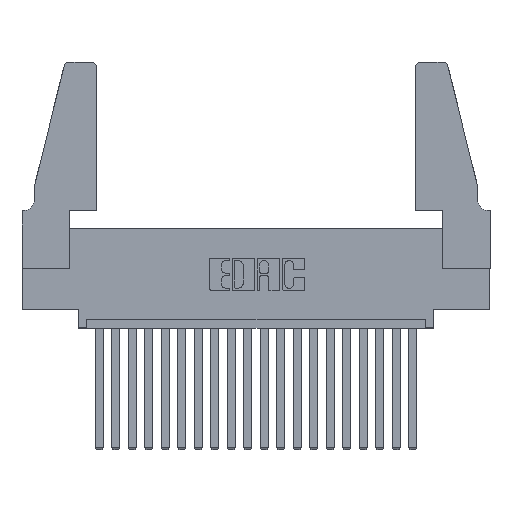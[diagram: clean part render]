
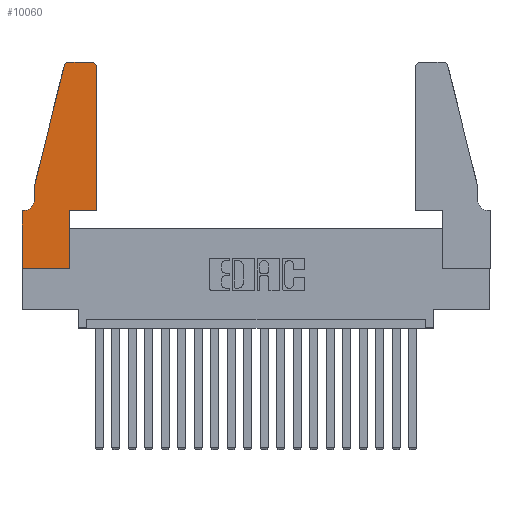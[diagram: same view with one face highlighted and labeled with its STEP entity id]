
A CAD part, top view. The second image highlights one B-rep face of the part: STEP entity #10060.
In plain terms, the highlighted planar face has unit normal (0, 0, 1).
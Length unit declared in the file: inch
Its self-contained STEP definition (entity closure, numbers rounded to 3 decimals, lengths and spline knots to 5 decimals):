
#19 = CARTESIAN_POINT ( 'NONE',  ( 0.0055, 0.42, 0.37 ) ) ;
#578 = CARTESIAN_POINT ( 'NONE',  ( 0.0055, 0.35, 0.37 ) ) ;
#1022 = VECTOR ( 'NONE', #19834, 39.37008 ) ;
#1233 = CARTESIAN_POINT ( 'NONE',  ( 0.2865, 0., 0.37 ) ) ;
#1356 = LINE ( 'NONE', #19567, #2580 ) ;
#1451 = ORIENTED_EDGE ( 'NONE', *, *, #14154, .T. ) ;
#1464 = CARTESIAN_POINT ( 'NONE',  ( 0.284, 1.22, 0.37 ) ) ;
#1550 = VERTEX_POINT ( 'NONE', #14343 ) ;
#1602 = DIRECTION ( 'NONE',  ( -1., 0., 0. ) ) ;
#1937 = EDGE_CURVE ( 'NONE', #1550, #16534, #11806, .T. ) ;
#1957 = FACE_OUTER_BOUND ( 'NONE', #10547, .T. ) ;
#2058 = CARTESIAN_POINT ( 'NONE',  ( 0.0755, 0.35, 0.37 ) ) ;
#2293 = VERTEX_POINT ( 'NONE', #10713 ) ;
#2319 = VERTEX_POINT ( 'NONE', #13852 ) ;
#2579 = VERTEX_POINT ( 'NONE', #9895 ) ;
#2580 = VECTOR ( 'NONE', #18085, 39.37008 ) ;
#2631 = AXIS2_PLACEMENT_3D ( 'NONE', #17480, #7623, #17284 ) ;
#2808 = DIRECTION ( 'NONE',  ( 0., -1., 0. ) ) ;
#2891 = AXIS2_PLACEMENT_3D ( 'NONE', #10846, #12426, #3139 ) ;
#2961 = EDGE_CURVE ( 'NONE', #15168, #2293, #11264, .T. ) ;
#2978 = LINE ( 'NONE', #6346, #14839 ) ;
#3139 = DIRECTION ( 'NONE',  ( 1., 0., 0. ) ) ;
#3312 = EDGE_CURVE ( 'NONE', #2579, #7679, #9764, .T. ) ;
#3616 = DIRECTION ( 'NONE',  ( -1., 0., 0. ) ) ;
#3888 = CIRCLE ( 'NONE', #12414, 0.07 ) ;
#4105 = DIRECTION ( 'NONE',  ( 1., 0., 0. ) ) ;
#4140 = CARTESIAN_POINT ( 'NONE',  ( 0.0755, 0.42, 0.37 ) ) ;
#4403 = CARTESIAN_POINT ( 'NONE',  ( 0.0755, 0.5, 0.37 ) ) ;
#5085 = PLANE ( 'NONE',  #2631 ) ;
#5205 = ORIENTED_EDGE ( 'NONE', *, *, #8197, .T. ) ;
#5272 = ORIENTED_EDGE ( 'NONE', *, *, #19831, .T. ) ;
#5373 = DIRECTION ( 'NONE',  ( -0.239, -0.971, 0. ) ) ;
#5595 = LINE ( 'NONE', #7720, #6585 ) ;
#5900 = ORIENTED_EDGE ( 'NONE', *, *, #10368, .T. ) ;
#5956 = CARTESIAN_POINT ( 'NONE',  ( 0.25487, 1.22718, 0.37 ) ) ;
#6346 = CARTESIAN_POINT ( 'NONE',  ( 0., 0., 0.37 ) ) ;
#6457 = VERTEX_POINT ( 'NONE', #1233 ) ;
#6569 = ORIENTED_EDGE ( 'NONE', *, *, #2961, .T. ) ;
#6585 = VECTOR ( 'NONE', #2808, 39.37008 ) ;
#7073 = DIRECTION ( 'NONE',  ( 0., 1., 0. ) ) ;
#7439 = VECTOR ( 'NONE', #4105, 39.37008 ) ;
#7531 = DIRECTION ( 'NONE',  ( 0., 0., 1. ) ) ;
#7623 = DIRECTION ( 'NONE',  ( 0., 0., 1. ) ) ;
#7666 = VECTOR ( 'NONE', #19336, 39.37008 ) ;
#7679 = VERTEX_POINT ( 'NONE', #5956 ) ;
#7720 = CARTESIAN_POINT ( 'NONE',  ( 0., 0., 0.37 ) ) ;
#7839 = VECTOR ( 'NONE', #7073, 39.37008 ) ;
#7987 = ORIENTED_EDGE ( 'NONE', *, *, #17327, .T. ) ;
#8197 = EDGE_CURVE ( 'NONE', #9604, #16167, #17577, .T. ) ;
#8325 = ORIENTED_EDGE ( 'NONE', *, *, #12683, .T. ) ;
#8541 = CARTESIAN_POINT ( 'NONE',  ( 0.4205, 1.25, 0.37 ) ) ;
#8798 = VERTEX_POINT ( 'NONE', #8541 ) ;
#8947 = CARTESIAN_POINT ( 'NONE',  ( 0.4505, 0.35, 0.37 ) ) ;
#9044 = ORIENTED_EDGE ( 'NONE', *, *, #18455, .T. ) ;
#9604 = VERTEX_POINT ( 'NONE', #13396 ) ;
#9764 = CIRCLE ( 'NONE', #10133, 0.03 ) ;
#9895 = CARTESIAN_POINT ( 'NONE',  ( 0.284, 1.25, 0.37 ) ) ;
#10060 = ADVANCED_FACE ( 'NONE', ( #1957 ), #5085, .T. ) ;
#10133 = AXIS2_PLACEMENT_3D ( 'NONE', #1464, #7531, #13584 ) ;
#10311 = EDGE_CURVE ( 'NONE', #2293, #16990, #5595, .T. ) ;
#10368 = EDGE_CURVE ( 'NONE', #8798, #2579, #1356, .T. ) ;
#10547 = EDGE_LOOP ( 'NONE', ( #5900, #13013, #8325, #16942, #9044, #6569, #11474, #7987, #11704, #5272, #5205, #1451 ) ) ;
#10713 = CARTESIAN_POINT ( 'NONE',  ( 0., 0.35, 0.37 ) ) ;
#10846 = CARTESIAN_POINT ( 'NONE',  ( 0.4205, 1.22, 0.37 ) ) ;
#10873 = DIRECTION ( 'NONE',  ( 0., 0., -1. ) ) ;
#11233 = CARTESIAN_POINT ( 'NONE',  ( 0., 0., 0.37 ) ) ;
#11264 = LINE ( 'NONE', #2058, #18071 ) ;
#11474 = ORIENTED_EDGE ( 'NONE', *, *, #10311, .T. ) ;
#11704 = ORIENTED_EDGE ( 'NONE', *, *, #14334, .T. ) ;
#11806 = LINE ( 'NONE', #4403, #7666 ) ;
#11831 = CARTESIAN_POINT ( 'NONE',  ( 0.4505, 0.35, 0.37 ) ) ;
#11990 = LINE ( 'NONE', #16453, #7839 ) ;
#12414 = AXIS2_PLACEMENT_3D ( 'NONE', #19, #10873, #1602 ) ;
#12426 = DIRECTION ( 'NONE',  ( 0., 0., 1. ) ) ;
#12515 = DIRECTION ( 'NONE',  ( 1., 0., 0. ) ) ;
#12683 = EDGE_CURVE ( 'NONE', #7679, #1550, #12772, .T. ) ;
#12772 = LINE ( 'NONE', #16264, #16683 ) ;
#13013 = ORIENTED_EDGE ( 'NONE', *, *, #3312, .T. ) ;
#13396 = CARTESIAN_POINT ( 'NONE',  ( 0.4505, 0.35, 0.37 ) ) ;
#13584 = DIRECTION ( 'NONE',  ( 1., 0., 0. ) ) ;
#13852 = CARTESIAN_POINT ( 'NONE',  ( 0.2865, 0.35, 0.37 ) ) ;
#14154 = EDGE_CURVE ( 'NONE', #16167, #8798, #18067, .T. ) ;
#14334 = EDGE_CURVE ( 'NONE', #6457, #2319, #11990, .T. ) ;
#14343 = CARTESIAN_POINT ( 'NONE',  ( 0.0755, 0.5, 0.37 ) ) ;
#14839 = VECTOR ( 'NONE', #12515, 39.37008 ) ;
#15168 = VERTEX_POINT ( 'NONE', #578 ) ;
#15530 = CARTESIAN_POINT ( 'NONE',  ( 0.4505, 1.22, 0.37 ) ) ;
#16167 = VERTEX_POINT ( 'NONE', #15530 ) ;
#16264 = CARTESIAN_POINT ( 'NONE',  ( 0.0755, 0.5, 0.37 ) ) ;
#16453 = CARTESIAN_POINT ( 'NONE',  ( 0.2865, 0.35, 0.37 ) ) ;
#16534 = VERTEX_POINT ( 'NONE', #4140 ) ;
#16683 = VECTOR ( 'NONE', #5373, 39.37008 ) ;
#16942 = ORIENTED_EDGE ( 'NONE', *, *, #1937, .T. ) ;
#16990 = VERTEX_POINT ( 'NONE', #11233 ) ;
#17284 = DIRECTION ( 'NONE',  ( 1., 0., 0. ) ) ;
#17327 = EDGE_CURVE ( 'NONE', #16990, #6457, #2978, .T. ) ;
#17480 = CARTESIAN_POINT ( 'NONE',  ( 0., 0.35, 0.37 ) ) ;
#17577 = LINE ( 'NONE', #8947, #1022 ) ;
#18067 = CIRCLE ( 'NONE', #2891, 0.03 ) ;
#18071 = VECTOR ( 'NONE', #3616, 39.37008 ) ;
#18085 = DIRECTION ( 'NONE',  ( -1., 0., 0. ) ) ;
#18455 = EDGE_CURVE ( 'NONE', #16534, #15168, #3888, .T. ) ;
#19336 = DIRECTION ( 'NONE',  ( 0., -1., 0. ) ) ;
#19567 = CARTESIAN_POINT ( 'NONE',  ( 0.2605, 1.25, 0.37 ) ) ;
#19831 = EDGE_CURVE ( 'NONE', #2319, #9604, #19853, .T. ) ;
#19834 = DIRECTION ( 'NONE',  ( 0., 1., 0. ) ) ;
#19853 = LINE ( 'NONE', #11831, #7439 ) ;
